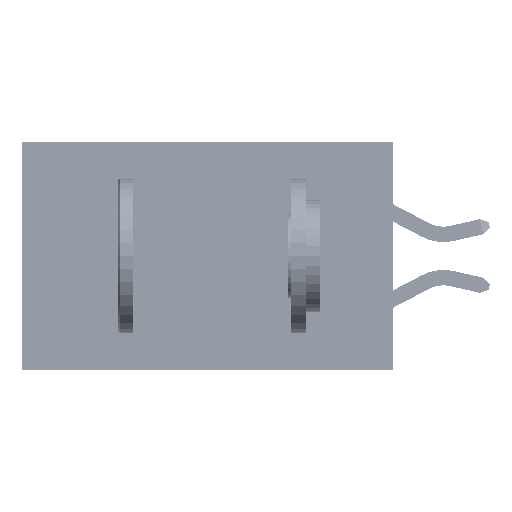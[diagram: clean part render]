
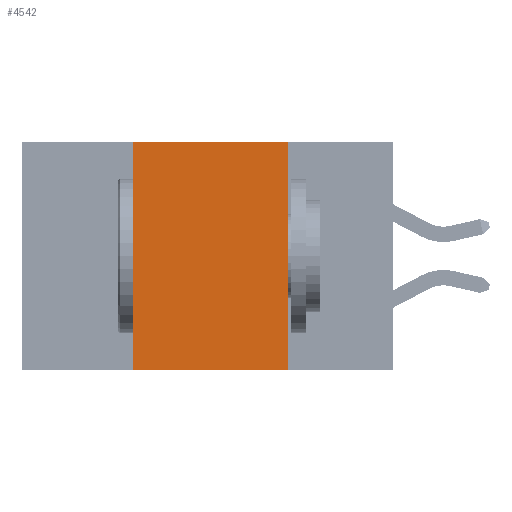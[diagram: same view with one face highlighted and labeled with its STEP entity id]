
A CAD part, left-side view. The second image highlights one B-rep face of the part: STEP entity #4542.
In plain terms, the highlighted planar face has unit normal (-1, 0, 0).
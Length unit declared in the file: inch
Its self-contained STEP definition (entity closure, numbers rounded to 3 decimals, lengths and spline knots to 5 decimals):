
#283 = CARTESIAN_POINT ( 'NONE',  ( 0., 0.6, -0.37 ) ) ;
#2418 = CARTESIAN_POINT ( 'NONE',  ( 0., 0.6, 0. ) ) ;
#3615 = CARTESIAN_POINT ( 'NONE',  ( 0., 0.17, 0. ) ) ;
#4542 = ADVANCED_FACE ( 'NONE', ( #44370 ), #7720, .F. ) ;
#4730 = EDGE_CURVE ( 'NONE', #21620, #13400, #44329, .T. ) ;
#5019 = EDGE_CURVE ( 'NONE', #5406, #12387, #23959, .T. ) ;
#5406 = VERTEX_POINT ( 'NONE', #14851 ) ;
#6941 = EDGE_LOOP ( 'NONE', ( #38451, #20946, #33191, #30306 ) ) ;
#7720 = PLANE ( 'NONE',  #13938 ) ;
#8914 = VECTOR ( 'NONE', #20659, 39.37008 ) ;
#10522 = VECTOR ( 'NONE', #26378, 39.37008 ) ;
#12387 = VERTEX_POINT ( 'NONE', #28735 ) ;
#13400 = VERTEX_POINT ( 'NONE', #41209 ) ;
#13938 = AXIS2_PLACEMENT_3D ( 'NONE', #41277, #27645, #31090 ) ;
#14851 = CARTESIAN_POINT ( 'NONE',  ( 0., 0.17, 0. ) ) ;
#15865 = EDGE_CURVE ( 'NONE', #13400, #5406, #29271, .T. ) ;
#17583 = VECTOR ( 'NONE', #19124, 39.37008 ) ;
#18046 = LINE ( 'NONE', #283, #8914 ) ;
#19124 = DIRECTION ( 'NONE',  ( 0., 0., 1. ) ) ;
#20559 = DIRECTION ( 'NONE',  ( 0., 0., -1. ) ) ;
#20659 = DIRECTION ( 'NONE',  ( 0., -1., 0. ) ) ;
#20946 = ORIENTED_EDGE ( 'NONE', *, *, #15865, .F. ) ;
#21620 = VERTEX_POINT ( 'NONE', #32315 ) ;
#23959 = LINE ( 'NONE', #3615, #31975 ) ;
#26250 = CARTESIAN_POINT ( 'NONE',  ( 0., 0.42, 0. ) ) ;
#26378 = DIRECTION ( 'NONE',  ( 0., -1., 0. ) ) ;
#27645 = DIRECTION ( 'NONE',  ( 1., 0., 0. ) ) ;
#28735 = CARTESIAN_POINT ( 'NONE',  ( 0., 0.17, -0.37 ) ) ;
#29271 = LINE ( 'NONE', #2418, #10522 ) ;
#30306 = ORIENTED_EDGE ( 'NONE', *, *, #35540, .T. ) ;
#31090 = DIRECTION ( 'NONE',  ( 0., 0., -1. ) ) ;
#31975 = VECTOR ( 'NONE', #20559, 39.37008 ) ;
#32315 = CARTESIAN_POINT ( 'NONE',  ( 0., 0.42, -0.37 ) ) ;
#33191 = ORIENTED_EDGE ( 'NONE', *, *, #4730, .F. ) ;
#35540 = EDGE_CURVE ( 'NONE', #21620, #12387, #18046, .T. ) ;
#38451 = ORIENTED_EDGE ( 'NONE', *, *, #5019, .F. ) ;
#41209 = CARTESIAN_POINT ( 'NONE',  ( 0., 0.42, 0. ) ) ;
#41277 = CARTESIAN_POINT ( 'NONE',  ( 0., 0.6, 0. ) ) ;
#44329 = LINE ( 'NONE', #26250, #17583 ) ;
#44370 = FACE_OUTER_BOUND ( 'NONE', #6941, .T. ) ;
